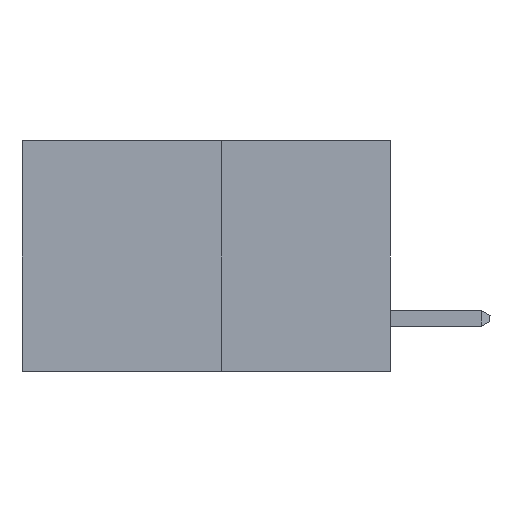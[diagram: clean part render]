
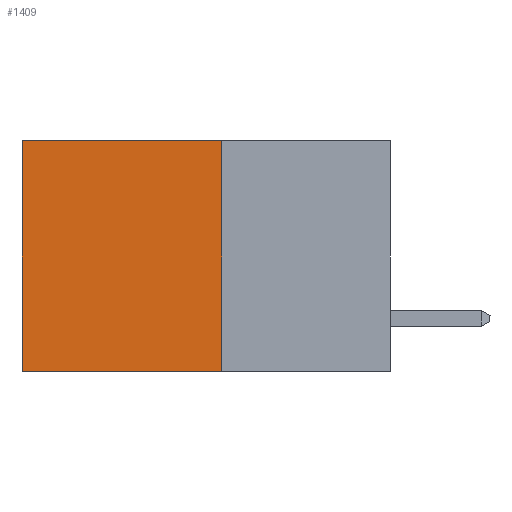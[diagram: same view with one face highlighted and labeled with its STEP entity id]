
A CAD part, left-side view. The second image highlights one B-rep face of the part: STEP entity #1409.
In plain terms, the highlighted planar face has unit normal (-1, 0, 0).
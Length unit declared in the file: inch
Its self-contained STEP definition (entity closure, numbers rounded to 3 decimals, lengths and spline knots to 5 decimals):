
#362 = LINE ( 'NONE', #2112, #5564 ) ;
#951 = ORIENTED_EDGE ( 'NONE', *, *, #7158, .T. ) ;
#1245 = ORIENTED_EDGE ( 'NONE', *, *, #10514, .F. ) ;
#1249 = CARTESIAN_POINT ( 'NONE',  ( 0.277, 0.59, -0.37 ) ) ;
#1405 = DIRECTION ( 'NONE',  ( 0., 0., -1. ) ) ;
#1409 = ADVANCED_FACE ( 'NONE', ( #12346 ), #4036, .F. ) ;
#2112 = CARTESIAN_POINT ( 'NONE',  ( 0.277, 0.27, 0. ) ) ;
#2508 = ORIENTED_EDGE ( 'NONE', *, *, #8106, .F. ) ;
#2701 = VERTEX_POINT ( 'NONE', #5566 ) ;
#2743 = CARTESIAN_POINT ( 'NONE',  ( 0.277, 0.27, -0.37 ) ) ;
#2908 = DIRECTION ( 'NONE',  ( 0., 1., 0. ) ) ;
#3450 = ORIENTED_EDGE ( 'NONE', *, *, #11800, .T. ) ;
#3602 = DIRECTION ( 'NONE',  ( 0., 0., -1. ) ) ;
#4036 = PLANE ( 'NONE',  #8712 ) ;
#4290 = CARTESIAN_POINT ( 'NONE',  ( 0.277, 0.27, 0. ) ) ;
#4304 = CARTESIAN_POINT ( 'NONE',  ( 0.277, 0.59, -0.37 ) ) ;
#4367 = DIRECTION ( 'NONE',  ( 0., 0., -1. ) ) ;
#4381 = DIRECTION ( 'NONE',  ( 1., 0., 0. ) ) ;
#5564 = VECTOR ( 'NONE', #6210, 39.37008 ) ;
#5566 = CARTESIAN_POINT ( 'NONE',  ( 0.277, 0.59, 0. ) ) ;
#5814 = EDGE_LOOP ( 'NONE', ( #951, #1245, #2508, #3450 ) ) ;
#6181 = VERTEX_POINT ( 'NONE', #4290 ) ;
#6210 = DIRECTION ( 'NONE',  ( 0., 1., 0. ) ) ;
#6298 = VECTOR ( 'NONE', #2908, 39.37008 ) ;
#6612 = VECTOR ( 'NONE', #3602, 39.37008 ) ;
#7158 = EDGE_CURVE ( 'NONE', #2701, #7874, #12324, .T. ) ;
#7351 = CARTESIAN_POINT ( 'NONE',  ( 0.277, 0.27, -0.37 ) ) ;
#7874 = VERTEX_POINT ( 'NONE', #4304 ) ;
#8106 = EDGE_CURVE ( 'NONE', #6181, #10893, #9249, .T. ) ;
#8606 = CARTESIAN_POINT ( 'NONE',  ( 0.277, 0.27, -0.37 ) ) ;
#8627 = LINE ( 'NONE', #9956, #6298 ) ;
#8712 = AXIS2_PLACEMENT_3D ( 'NONE', #7351, #4381, #4367 ) ;
#9249 = LINE ( 'NONE', #8606, #6612 ) ;
#9733 = VECTOR ( 'NONE', #1405, 39.37008 ) ;
#9956 = CARTESIAN_POINT ( 'NONE',  ( 0.277, 0.27, -0.37 ) ) ;
#10514 = EDGE_CURVE ( 'NONE', #10893, #7874, #8627, .T. ) ;
#10893 = VERTEX_POINT ( 'NONE', #2743 ) ;
#11800 = EDGE_CURVE ( 'NONE', #6181, #2701, #362, .T. ) ;
#12324 = LINE ( 'NONE', #1249, #9733 ) ;
#12346 = FACE_OUTER_BOUND ( 'NONE', #5814, .T. ) ;
